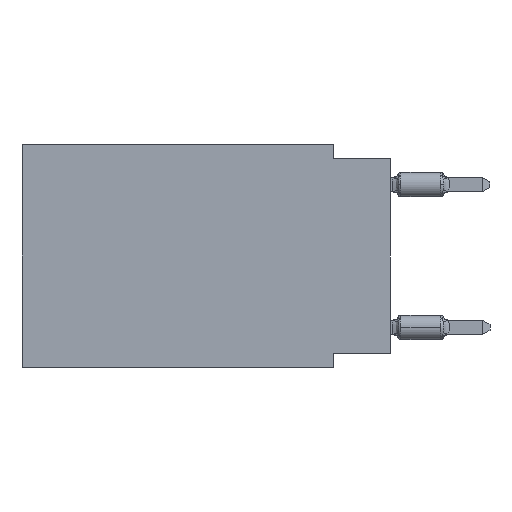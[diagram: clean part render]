
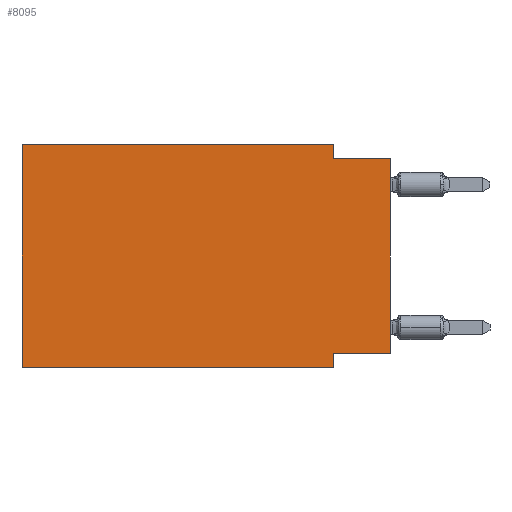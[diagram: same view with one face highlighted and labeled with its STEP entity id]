
A CAD part, left-side view. The second image highlights one B-rep face of the part: STEP entity #8095.
In plain terms, the highlighted planar face has unit normal (-1, 0, 0).
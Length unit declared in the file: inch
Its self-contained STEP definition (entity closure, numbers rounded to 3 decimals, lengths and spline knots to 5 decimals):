
#982 = CARTESIAN_POINT ( 'NONE',  ( 0., 0.1, -0.39 ) ) ;
#997 = CARTESIAN_POINT ( 'NONE',  ( 0., 0.645, -0.39 ) ) ;
#1165 = ORIENTED_EDGE ( 'NONE', *, *, #4105, .F. ) ;
#1385 = ORIENTED_EDGE ( 'NONE', *, *, #24119, .T. ) ;
#1450 = LINE ( 'NONE', #16377, #7920 ) ;
#1850 = EDGE_CURVE ( 'NONE', #17483, #19424, #8973, .T. ) ;
#1935 = DIRECTION ( 'NONE',  ( 0., 0., 1. ) ) ;
#2428 = EDGE_CURVE ( 'NONE', #27130, #2919, #26967, .T. ) ;
#2560 = LINE ( 'NONE', #4583, #13570 ) ;
#2919 = VERTEX_POINT ( 'NONE', #9569 ) ;
#3525 = ORIENTED_EDGE ( 'NONE', *, *, #4160, .T. ) ;
#3836 = ORIENTED_EDGE ( 'NONE', *, *, #2428, .F. ) ;
#3840 = EDGE_LOOP ( 'NONE', ( #1385, #25406, #3836, #1165, #20484, #3525, #21370, #18426 ) ) ;
#4105 = EDGE_CURVE ( 'NONE', #16676, #27130, #7550, .T. ) ;
#4160 = EDGE_CURVE ( 'NONE', #7489, #19424, #27790, .T. ) ;
#4583 = CARTESIAN_POINT ( 'NONE',  ( 0., 0., -0.365 ) ) ;
#4805 = VECTOR ( 'NONE', #9254, 39.37008 ) ;
#4885 = CARTESIAN_POINT ( 'NONE',  ( 0., 0.645, 0. ) ) ;
#7080 = EDGE_CURVE ( 'NONE', #2919, #21824, #1450, .T. ) ;
#7402 = CARTESIAN_POINT ( 'NONE',  ( 0., 0.645, -0.39 ) ) ;
#7489 = VERTEX_POINT ( 'NONE', #997 ) ;
#7550 = LINE ( 'NONE', #14496, #13367 ) ;
#7920 = VECTOR ( 'NONE', #16658, 39.37008 ) ;
#8095 = ADVANCED_FACE ( 'NONE', ( #11734 ), #24775, .F. ) ;
#8973 = LINE ( 'NONE', #17821, #4805 ) ;
#9031 = EDGE_CURVE ( 'NONE', #24000, #17483, #2560, .T. ) ;
#9078 = CARTESIAN_POINT ( 'NONE',  ( 0., 0., -0.365 ) ) ;
#9235 = VECTOR ( 'NONE', #1935, 39.37008 ) ;
#9254 = DIRECTION ( 'NONE',  ( 0., 0., -1. ) ) ;
#9275 = DIRECTION ( 'NONE',  ( 0., 0., -1. ) ) ;
#9569 = CARTESIAN_POINT ( 'NONE',  ( 0., 0.1, -0.025 ) ) ;
#9574 = DIRECTION ( 'NONE',  ( 0., -1., 0. ) ) ;
#9697 = CARTESIAN_POINT ( 'NONE',  ( 0., 0.645, 0. ) ) ;
#10116 = VECTOR ( 'NONE', #25203, 39.37008 ) ;
#11056 = CARTESIAN_POINT ( 'NONE',  ( 0., 0.1, 0. ) ) ;
#11734 = FACE_OUTER_BOUND ( 'NONE', #3840, .T. ) ;
#11823 = DIRECTION ( 'NONE',  ( 0., 0., 1. ) ) ;
#11884 = DIRECTION ( 'NONE',  ( 1., 0., 0. ) ) ;
#12361 = LINE ( 'NONE', #21194, #9235 ) ;
#13367 = VECTOR ( 'NONE', #9574, 39.37008 ) ;
#13417 = DIRECTION ( 'NONE',  ( 0., 1., 0. ) ) ;
#13570 = VECTOR ( 'NONE', #13417, 39.37008 ) ;
#14496 = CARTESIAN_POINT ( 'NONE',  ( 0., 0.645, 0. ) ) ;
#16377 = CARTESIAN_POINT ( 'NONE',  ( 0., 0., -0.025 ) ) ;
#16612 = CARTESIAN_POINT ( 'NONE',  ( 0., 0.1, -0.365 ) ) ;
#16658 = DIRECTION ( 'NONE',  ( 0., -1., 0. ) ) ;
#16676 = VERTEX_POINT ( 'NONE', #18998 ) ;
#17483 = VERTEX_POINT ( 'NONE', #16612 ) ;
#17821 = CARTESIAN_POINT ( 'NONE',  ( 0., 0.1, -0.39 ) ) ;
#18166 = DIRECTION ( 'NONE',  ( 0., 0., -1. ) ) ;
#18329 = VECTOR ( 'NONE', #11823, 39.37008 ) ;
#18426 = ORIENTED_EDGE ( 'NONE', *, *, #9031, .F. ) ;
#18998 = CARTESIAN_POINT ( 'NONE',  ( 0., 0.645, 0. ) ) ;
#19424 = VERTEX_POINT ( 'NONE', #982 ) ;
#19507 = EDGE_CURVE ( 'NONE', #7489, #16676, #24723, .T. ) ;
#20484 = ORIENTED_EDGE ( 'NONE', *, *, #19507, .F. ) ;
#20566 = VECTOR ( 'NONE', #18166, 39.37008 ) ;
#21194 = CARTESIAN_POINT ( 'NONE',  ( 0., 0., 0. ) ) ;
#21370 = ORIENTED_EDGE ( 'NONE', *, *, #1850, .F. ) ;
#21824 = VERTEX_POINT ( 'NONE', #27340 ) ;
#24000 = VERTEX_POINT ( 'NONE', #9078 ) ;
#24119 = EDGE_CURVE ( 'NONE', #24000, #21824, #12361, .T. ) ;
#24679 = CARTESIAN_POINT ( 'NONE',  ( 0., 0.1, 0. ) ) ;
#24723 = LINE ( 'NONE', #4885, #18329 ) ;
#24775 = PLANE ( 'NONE',  #26907 ) ;
#25203 = DIRECTION ( 'NONE',  ( 0., -1., 0. ) ) ;
#25406 = ORIENTED_EDGE ( 'NONE', *, *, #7080, .F. ) ;
#26907 = AXIS2_PLACEMENT_3D ( 'NONE', #9697, #11884, #9275 ) ;
#26967 = LINE ( 'NONE', #24679, #20566 ) ;
#27130 = VERTEX_POINT ( 'NONE', #11056 ) ;
#27340 = CARTESIAN_POINT ( 'NONE',  ( 0., 0., -0.025 ) ) ;
#27790 = LINE ( 'NONE', #7402, #10116 ) ;
